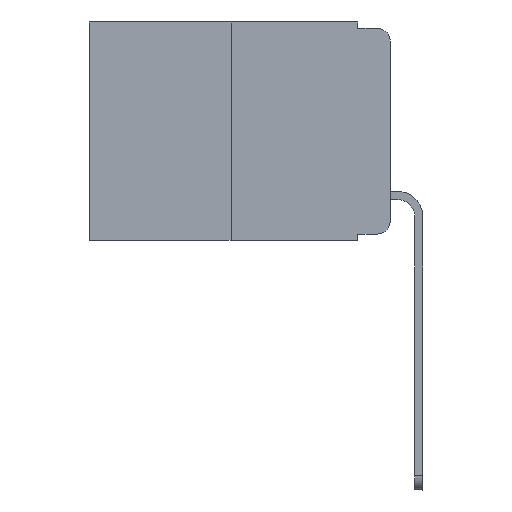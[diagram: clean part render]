
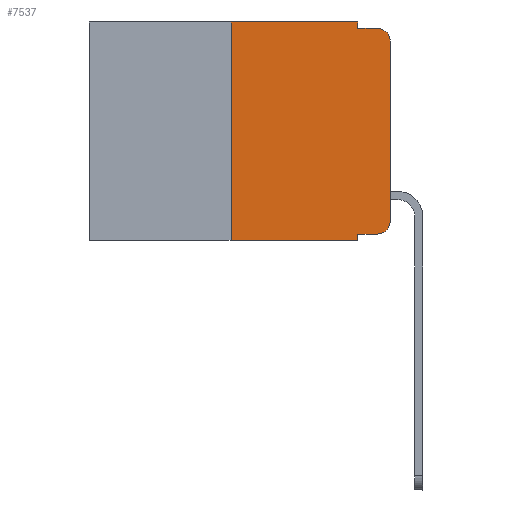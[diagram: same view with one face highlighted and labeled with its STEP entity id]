
A CAD part, left-side view. The second image highlights one B-rep face of the part: STEP entity #7537.
In plain terms, the highlighted planar face has unit normal (-1, 0, 0).
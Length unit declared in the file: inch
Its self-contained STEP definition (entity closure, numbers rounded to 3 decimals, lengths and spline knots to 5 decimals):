
#44 = CARTESIAN_POINT ( 'NONE',  ( 0., 0., -0.313 ) ) ;
#610 = ORIENTED_EDGE ( 'NONE', *, *, #15861, .F. ) ;
#615 = LINE ( 'NONE', #6234, #5508 ) ;
#622 = VERTEX_POINT ( 'NONE', #12190 ) ;
#1029 = DIRECTION ( 'NONE',  ( 0., -1., 0. ) ) ;
#1350 = VECTOR ( 'NONE', #17337, 39.37008 ) ;
#1595 = EDGE_CURVE ( 'NONE', #15957, #5804, #13634, .T. ) ;
#2261 = CARTESIAN_POINT ( 'NONE',  ( 0., 0., 0. ) ) ;
#3036 = CARTESIAN_POINT ( 'NONE',  ( 0., 0.02, -0.313 ) ) ;
#3455 = EDGE_LOOP ( 'NONE', ( #9517, #13168, #18147, #8723, #9699, #11393, #4524, #610, #13750, #9004 ) ) ;
#3469 = VERTEX_POINT ( 'NONE', #16932 ) ;
#3925 = LINE ( 'NONE', #13944, #12244 ) ;
#4139 = EDGE_CURVE ( 'NONE', #7986, #3469, #14958, .T. ) ;
#4524 = ORIENTED_EDGE ( 'NONE', *, *, #11237, .T. ) ;
#4817 = DIRECTION ( 'NONE',  ( 1., 0., 0. ) ) ;
#5400 = DIRECTION ( 'NONE',  ( 0., -1., 0. ) ) ;
#5508 = VECTOR ( 'NONE', #10436, 39.37008 ) ;
#5664 = EDGE_CURVE ( 'NONE', #5718, #3469, #12652, .T. ) ;
#5718 = VERTEX_POINT ( 'NONE', #16907 ) ;
#5769 = DIRECTION ( 'NONE',  ( 0., 0., -1. ) ) ;
#5804 = VERTEX_POINT ( 'NONE', #11545 ) ;
#6007 = EDGE_CURVE ( 'NONE', #11267, #5718, #16864, .T. ) ;
#6112 = LINE ( 'NONE', #6282, #1350 ) ;
#6199 = CARTESIAN_POINT ( 'NONE',  ( 0., 0.473, 0. ) ) ;
#6234 = CARTESIAN_POINT ( 'NONE',  ( 0., 0.051, 0. ) ) ;
#6282 = CARTESIAN_POINT ( 'NONE',  ( 0., 0.25, 0. ) ) ;
#6462 = VECTOR ( 'NONE', #12994, 39.37008 ) ;
#6775 = CARTESIAN_POINT ( 'NONE',  ( 0., 0.051, -0.343 ) ) ;
#7056 = DIRECTION ( 'NONE',  ( -1., 0., 0. ) ) ;
#7172 = CARTESIAN_POINT ( 'NONE',  ( 0., 0.25, -0.343 ) ) ;
#7328 = CIRCLE ( 'NONE', #14733, 0.02 ) ;
#7537 = ADVANCED_FACE ( 'NONE', ( #13186 ), #10142, .F. ) ;
#7940 = CARTESIAN_POINT ( 'NONE',  ( 0., 0.051, -0.01 ) ) ;
#7986 = VERTEX_POINT ( 'NONE', #13419 ) ;
#8580 = CARTESIAN_POINT ( 'NONE',  ( 0., 0.051, 0. ) ) ;
#8621 = EDGE_CURVE ( 'NONE', #16125, #622, #6112, .T. ) ;
#8723 = ORIENTED_EDGE ( 'NONE', *, *, #11057, .F. ) ;
#8804 = CARTESIAN_POINT ( 'NONE',  ( 0., 0.473, 0. ) ) ;
#8844 = DIRECTION ( 'NONE',  ( 0., 0., -1. ) ) ;
#9004 = ORIENTED_EDGE ( 'NONE', *, *, #13667, .T. ) ;
#9517 = ORIENTED_EDGE ( 'NONE', *, *, #6007, .T. ) ;
#9586 = VERTEX_POINT ( 'NONE', #6775 ) ;
#9699 = ORIENTED_EDGE ( 'NONE', *, *, #17221, .F. ) ;
#10142 = PLANE ( 'NONE',  #12465 ) ;
#10436 = DIRECTION ( 'NONE',  ( 0., 0., -1. ) ) ;
#11057 = EDGE_CURVE ( 'NONE', #12490, #7986, #615, .T. ) ;
#11237 = EDGE_CURVE ( 'NONE', #16125, #9586, #3925, .T. ) ;
#11267 = VERTEX_POINT ( 'NONE', #44 ) ;
#11393 = ORIENTED_EDGE ( 'NONE', *, *, #8621, .F. ) ;
#11545 = CARTESIAN_POINT ( 'NONE',  ( 0., 0.02, -0.333 ) ) ;
#11930 = VECTOR ( 'NONE', #1029, 39.37008 ) ;
#12190 = CARTESIAN_POINT ( 'NONE',  ( 0., 0.25, 0. ) ) ;
#12244 = VECTOR ( 'NONE', #5400, 39.37008 ) ;
#12465 = AXIS2_PLACEMENT_3D ( 'NONE', #6199, #4817, #8844 ) ;
#12490 = VERTEX_POINT ( 'NONE', #8580 ) ;
#12652 = CIRCLE ( 'NONE', #16506, 0.02 ) ;
#12903 = LINE ( 'NONE', #15757, #6462 ) ;
#12994 = DIRECTION ( 'NONE',  ( 0., 0., -1. ) ) ;
#13168 = ORIENTED_EDGE ( 'NONE', *, *, #5664, .T. ) ;
#13186 = FACE_OUTER_BOUND ( 'NONE', #3455, .T. ) ;
#13419 = CARTESIAN_POINT ( 'NONE',  ( 0., 0.051, -0.01 ) ) ;
#13579 = DIRECTION ( 'NONE',  ( 0., -1., 0. ) ) ;
#13634 = LINE ( 'NONE', #15296, #11930 ) ;
#13667 = EDGE_CURVE ( 'NONE', #5804, #11267, #7328, .T. ) ;
#13750 = ORIENTED_EDGE ( 'NONE', *, *, #1595, .T. ) ;
#13796 = VECTOR ( 'NONE', #15471, 39.37008 ) ;
#13944 = CARTESIAN_POINT ( 'NONE',  ( 0., 0.473, -0.343 ) ) ;
#14453 = VECTOR ( 'NONE', #17475, 39.37008 ) ;
#14559 = CARTESIAN_POINT ( 'NONE',  ( 0., 0.051, -0.333 ) ) ;
#14733 = AXIS2_PLACEMENT_3D ( 'NONE', #3036, #7056, #5769 ) ;
#14958 = LINE ( 'NONE', #7940, #15824 ) ;
#15165 = DIRECTION ( 'NONE',  ( 0., 0., -1. ) ) ;
#15296 = CARTESIAN_POINT ( 'NONE',  ( 0., 0.051, -0.333 ) ) ;
#15471 = DIRECTION ( 'NONE',  ( 0., 0., 1. ) ) ;
#15757 = CARTESIAN_POINT ( 'NONE',  ( 0., 0.051, 0. ) ) ;
#15824 = VECTOR ( 'NONE', #13579, 39.37008 ) ;
#15861 = EDGE_CURVE ( 'NONE', #15957, #9586, #12903, .T. ) ;
#15957 = VERTEX_POINT ( 'NONE', #14559 ) ;
#16125 = VERTEX_POINT ( 'NONE', #7172 ) ;
#16285 = LINE ( 'NONE', #8804, #14453 ) ;
#16506 = AXIS2_PLACEMENT_3D ( 'NONE', #16735, #17820, #15165 ) ;
#16735 = CARTESIAN_POINT ( 'NONE',  ( 0., 0.02, -0.03 ) ) ;
#16864 = LINE ( 'NONE', #2261, #13796 ) ;
#16907 = CARTESIAN_POINT ( 'NONE',  ( 0., 0., -0.03 ) ) ;
#16932 = CARTESIAN_POINT ( 'NONE',  ( 0., 0.02, -0.01 ) ) ;
#17221 = EDGE_CURVE ( 'NONE', #622, #12490, #16285, .T. ) ;
#17337 = DIRECTION ( 'NONE',  ( 0., 0., 1. ) ) ;
#17475 = DIRECTION ( 'NONE',  ( 0., -1., 0. ) ) ;
#17820 = DIRECTION ( 'NONE',  ( -1., 0., 0. ) ) ;
#18147 = ORIENTED_EDGE ( 'NONE', *, *, #4139, .F. ) ;
